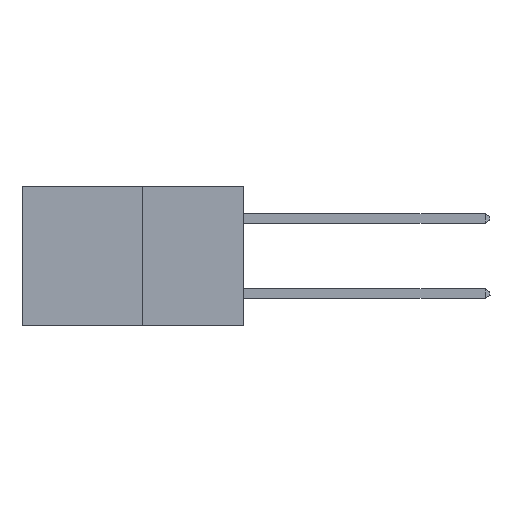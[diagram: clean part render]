
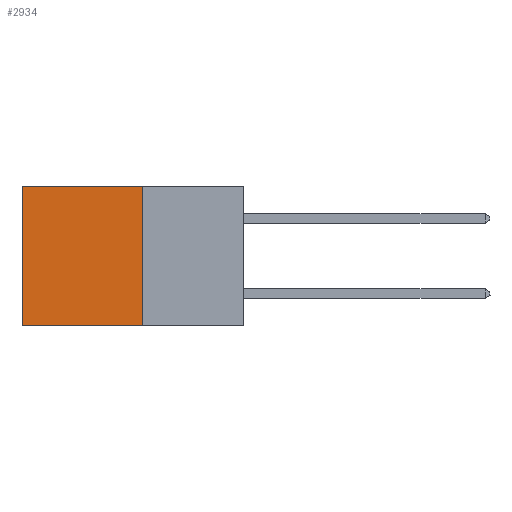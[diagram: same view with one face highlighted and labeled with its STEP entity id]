
A CAD part, left-side view. The second image highlights one B-rep face of the part: STEP entity #2934.
In plain terms, the highlighted planar face has unit normal (-1, 0, 0).
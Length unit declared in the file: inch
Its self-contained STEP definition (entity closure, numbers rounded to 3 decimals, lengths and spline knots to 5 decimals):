
#169 = LINE ( 'NONE', #5957, #4479 ) ;
#387 = EDGE_CURVE ( 'NONE', #7921, #9443, #169, .T. ) ;
#506 = VERTEX_POINT ( 'NONE', #3071 ) ;
#1147 = CARTESIAN_POINT ( 'NONE',  ( 0.277, 0.27, -0.37 ) ) ;
#1291 = DIRECTION ( 'NONE',  ( 1., 0., 0. ) ) ;
#1866 = CARTESIAN_POINT ( 'NONE',  ( 0.277, 0.27, -0.37 ) ) ;
#2300 = LINE ( 'NONE', #8731, #4008 ) ;
#2371 = DIRECTION ( 'NONE',  ( 0., 0., -1. ) ) ;
#2398 = VECTOR ( 'NONE', #2371, 39.37008 ) ;
#2413 = CARTESIAN_POINT ( 'NONE',  ( 0.277, 0.59, -0.37 ) ) ;
#2934 = ADVANCED_FACE ( 'NONE', ( #6164 ), #9684, .F. ) ;
#3071 = CARTESIAN_POINT ( 'NONE',  ( 0.277, 0.27, 0. ) ) ;
#4008 = VECTOR ( 'NONE', #8623, 39.37008 ) ;
#4030 = DIRECTION ( 'NONE',  ( 0., 0., -1. ) ) ;
#4176 = EDGE_LOOP ( 'NONE', ( #4992, #5067, #5093, #5130 ) ) ;
#4181 = CARTESIAN_POINT ( 'NONE',  ( 0.277, 0.27, -0.37 ) ) ;
#4268 = EDGE_CURVE ( 'NONE', #506, #7921, #5399, .T. ) ;
#4479 = VECTOR ( 'NONE', #5483, 39.37008 ) ;
#4907 = CARTESIAN_POINT ( 'NONE',  ( 0.277, 0.59, -0.37 ) ) ;
#4992 = ORIENTED_EDGE ( 'NONE', *, *, #7670, .T. ) ;
#5067 = ORIENTED_EDGE ( 'NONE', *, *, #387, .F. ) ;
#5093 = ORIENTED_EDGE ( 'NONE', *, *, #4268, .F. ) ;
#5130 = ORIENTED_EDGE ( 'NONE', *, *, #6256, .T. ) ;
#5399 = LINE ( 'NONE', #4181, #9216 ) ;
#5483 = DIRECTION ( 'NONE',  ( 0., 1., 0. ) ) ;
#5957 = CARTESIAN_POINT ( 'NONE',  ( 0.277, 0.27, -0.37 ) ) ;
#5962 = DIRECTION ( 'NONE',  ( 0., 0., -1. ) ) ;
#6164 = FACE_OUTER_BOUND ( 'NONE', #4176, .T. ) ;
#6256 = EDGE_CURVE ( 'NONE', #506, #6598, #2300, .T. ) ;
#6598 = VERTEX_POINT ( 'NONE', #6998 ) ;
#6998 = CARTESIAN_POINT ( 'NONE',  ( 0.277, 0.59, 0. ) ) ;
#7670 = EDGE_CURVE ( 'NONE', #6598, #9443, #10009, .T. ) ;
#7921 = VERTEX_POINT ( 'NONE', #1147 ) ;
#8623 = DIRECTION ( 'NONE',  ( 0., 1., 0. ) ) ;
#8731 = CARTESIAN_POINT ( 'NONE',  ( 0.277, 0.27, 0. ) ) ;
#9216 = VECTOR ( 'NONE', #4030, 39.37008 ) ;
#9443 = VERTEX_POINT ( 'NONE', #4907 ) ;
#9623 = AXIS2_PLACEMENT_3D ( 'NONE', #1866, #1291, #5962 ) ;
#9684 = PLANE ( 'NONE',  #9623 ) ;
#10009 = LINE ( 'NONE', #2413, #2398 ) ;
